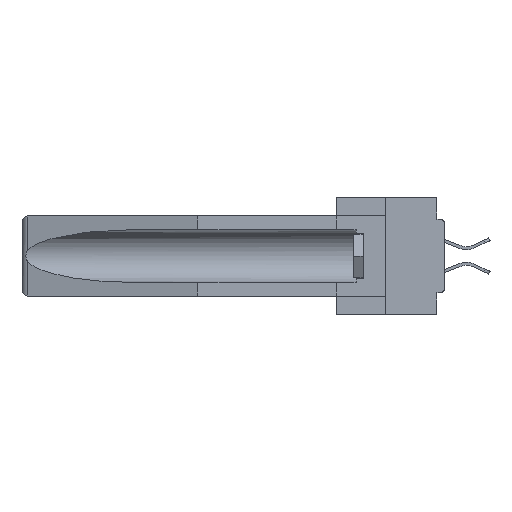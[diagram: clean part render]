
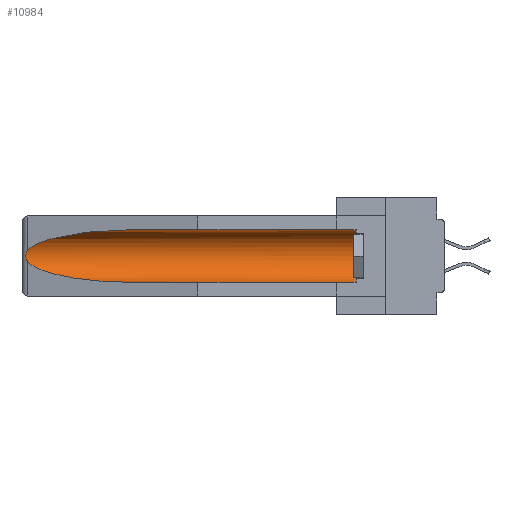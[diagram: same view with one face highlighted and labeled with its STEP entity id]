
A CAD part, left-side view. The second image highlights one B-rep face of the part: STEP entity #10984.
In plain terms, the highlighted cylindrical face has radius 2.857 mm (diameter 5.715 mm), a partial arc.
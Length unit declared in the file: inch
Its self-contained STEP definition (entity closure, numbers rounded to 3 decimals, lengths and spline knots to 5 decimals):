
#715 = DIRECTION ( 'NONE',  ( 0., 1., 0. ) ) ;
#1024 = EDGE_LOOP ( 'NONE', ( #7587, #22142, #10782, #5704, #25059, #8065 ) ) ;
#2954 = CARTESIAN_POINT ( 'NONE',  ( 0.155, -0.30754, -0.059 ) ) ;
#5041 = CARTESIAN_POINT ( 'NONE',  ( 0.26655, 1.53094, -0.18657 ) ) ;
#5083 = CARTESIAN_POINT ( 'NONE',  ( 0.26537, 1.52718, -0.19328 ) ) ;
#5704 = ORIENTED_EDGE ( 'NONE', *, *, #27604, .F. ) ;
#5762 = LINE ( 'NONE', #2954, #33327 ) ;
#5897 = CARTESIAN_POINT ( 'NONE',  ( 0.21114, 1.30732, -0.284 ) ) ;
#6249 = DIRECTION ( 'NONE',  ( 0., 1., 0. ) ) ;
#6546 = CIRCLE ( 'NONE', #23462, 0.1125 ) ;
#7208 = CARTESIAN_POINT ( 'NONE',  ( 0.26654, 1.53092, -0.15636 ) ) ;
#7587 = ORIENTED_EDGE ( 'NONE', *, *, #19947, .T. ) ;
#8065 = ORIENTED_EDGE ( 'NONE', *, *, #13815, .T. ) ;
#9135 = DIRECTION ( 'NONE',  ( 0., 0., 1. ) ) ;
#9443 = VERTEX_POINT ( 'NONE', #22329 ) ;
#10351 = CARTESIAN_POINT ( 'NONE',  ( 0.21114, 1.30732, -0.059 ) ) ;
#10716 =( BOUNDED_CURVE ( )  B_SPLINE_CURVE ( 3, ( #34923, #10351, #32228, #34559 ),
 .UNSPECIFIED., .F., .F. ) 
 B_SPLINE_CURVE_WITH_KNOTS ( ( 4, 4 ),
 ( 4.71239, 6.08839 ),
 .UNSPECIFIED. ) 
 CURVE ( )  GEOMETRIC_REPRESENTATION_ITEM ( )  RATIONAL_B_SPLINE_CURVE ( ( 1., 0.848, 0.848, 1. ) ) 
 REPRESENTATION_ITEM ( '' )  );
#10782 = ORIENTED_EDGE ( 'NONE', *, *, #20973, .T. ) ;
#10984 = ADVANCED_FACE ( 'NONE', ( #13486 ), #26417, .F. ) ;
#11850 = EDGE_CURVE ( 'NONE', #9443, #30042, #6546, .T. ) ;
#12555 = CARTESIAN_POINT ( 'NONE',  ( 0.26537, 1.52718, -0.14972 ) ) ;
#12747 = CARTESIAN_POINT ( 'NONE',  ( 0.2673, 1.5327, -0.16383 ) ) ;
#13453 = CARTESIAN_POINT ( 'NONE',  ( 0.26537, 1.52718, -0.19328 ) ) ;
#13486 = FACE_OUTER_BOUND ( 'NONE', #1024, .T. ) ;
#13496 = CARTESIAN_POINT ( 'NONE',  ( 0.25451, 1.48313, -0.24835 ) ) ;
#13815 = EDGE_CURVE ( 'NONE', #30042, #15106, #5762, .T. ) ;
#13948 = CARTESIAN_POINT ( 'NONE',  ( 0.155, 1.07973, -0.059 ) ) ;
#14770 = DIRECTION ( 'NONE',  ( 0., -1., 0. ) ) ;
#15106 = VERTEX_POINT ( 'NONE', #13948 ) ;
#17295 = VERTEX_POINT ( 'NONE', #33298 ) ;
#17689 = LINE ( 'NONE', #18636, #34027 ) ;
#18636 = CARTESIAN_POINT ( 'NONE',  ( 0.155, -0.30754, -0.284 ) ) ;
#19276 = AXIS2_PLACEMENT_3D ( 'NONE', #19863, #6249, #9135 ) ;
#19863 = CARTESIAN_POINT ( 'NONE',  ( 0.155, -0.30754, -0.1715 ) ) ;
#19947 = EDGE_CURVE ( 'NONE', #15106, #26967, #10716, .T. ) ;
#20973 = EDGE_CURVE ( 'NONE', #22201, #17295, #34759, .T. ) ;
#22142 = ORIENTED_EDGE ( 'NONE', *, *, #22542, .T. ) ;
#22201 = VERTEX_POINT ( 'NONE', #32138 ) ;
#22329 = CARTESIAN_POINT ( 'NONE',  ( 0.155, 0.126, -0.284 ) ) ;
#22542 = EDGE_CURVE ( 'NONE', #26967, #22201, #30869, .T. ) ;
#23462 = AXIS2_PLACEMENT_3D ( 'NONE', #25959, #14770, #28745 ) ;
#23725 = CARTESIAN_POINT ( 'NONE',  ( 0.26597, 1.52961, -0.15275 ) ) ;
#24309 = CARTESIAN_POINT ( 'NONE',  ( 0.26597, 1.5296, -0.19026 ) ) ;
#24687 = CARTESIAN_POINT ( 'NONE',  ( 0.155, 1.07973, -0.284 ) ) ;
#25059 = ORIENTED_EDGE ( 'NONE', *, *, #11850, .T. ) ;
#25959 = CARTESIAN_POINT ( 'NONE',  ( 0.155, 0.126, -0.1715 ) ) ;
#26417 = CYLINDRICAL_SURFACE ( 'NONE', #19276, 0.1125 ) ;
#26962 = CARTESIAN_POINT ( 'NONE',  ( 0.2673, 1.53269, -0.17917 ) ) ;
#26967 = VERTEX_POINT ( 'NONE', #12555 ) ;
#27067 = DIRECTION ( 'NONE',  ( 0., 1., 0. ) ) ;
#27205 = CARTESIAN_POINT ( 'NONE',  ( 0.2675, 1.53308, -0.17534 ) ) ;
#27604 = EDGE_CURVE ( 'NONE', #9443, #17295, #17689, .T. ) ;
#28745 = DIRECTION ( 'NONE',  ( 0., 0., 1. ) ) ;
#29120 = CARTESIAN_POINT ( 'NONE',  ( 0.155, 0.126, -0.059 ) ) ;
#30042 = VERTEX_POINT ( 'NONE', #29120 ) ;
#30869 = B_SPLINE_CURVE_WITH_KNOTS ( 'NONE', 3,
 ( #32097, #23725, #7208, #12747, #35167, #27205, #26962, #5041, #24309, #13453 ),
 .UNSPECIFIED., .F., .F.,
 ( 4, 2, 2, 2, 4 ),
 ( 0., 0.00029, 0.00058, 0.00087, 0.00117 ),
 .UNSPECIFIED. ) ;
#32097 = CARTESIAN_POINT ( 'NONE',  ( 0.26537, 1.52718, -0.14972 ) ) ;
#32138 = CARTESIAN_POINT ( 'NONE',  ( 0.26537, 1.52718, -0.19328 ) ) ;
#32228 = CARTESIAN_POINT ( 'NONE',  ( 0.25451, 1.48313, -0.09465 ) ) ;
#33298 = CARTESIAN_POINT ( 'NONE',  ( 0.155, 1.07973, -0.284 ) ) ;
#33327 = VECTOR ( 'NONE', #715, 39.37008 ) ;
#34027 = VECTOR ( 'NONE', #27067, 39.37008 ) ;
#34559 = CARTESIAN_POINT ( 'NONE',  ( 0.26537, 1.52718, -0.14972 ) ) ;
#34759 =( BOUNDED_CURVE ( )  B_SPLINE_CURVE ( 3, ( #5083, #13496, #5897, #24687 ),
 .UNSPECIFIED., .F., .F. ) 
 B_SPLINE_CURVE_WITH_KNOTS ( ( 4, 4 ),
 ( 0.1948, 1.5708 ),
 .UNSPECIFIED. ) 
 CURVE ( )  GEOMETRIC_REPRESENTATION_ITEM ( )  RATIONAL_B_SPLINE_CURVE ( ( 1., 0.848, 0.848, 1. ) ) 
 REPRESENTATION_ITEM ( '' )  );
#34923 = CARTESIAN_POINT ( 'NONE',  ( 0.155, 1.07973, -0.059 ) ) ;
#35167 = CARTESIAN_POINT ( 'NONE',  ( 0.2675, 1.53308, -0.16763 ) ) ;
